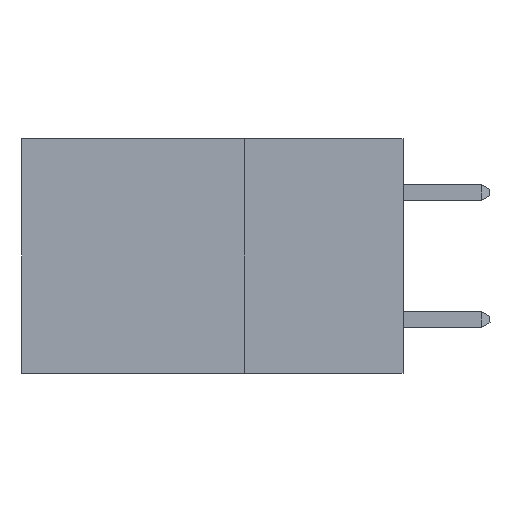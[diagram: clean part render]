
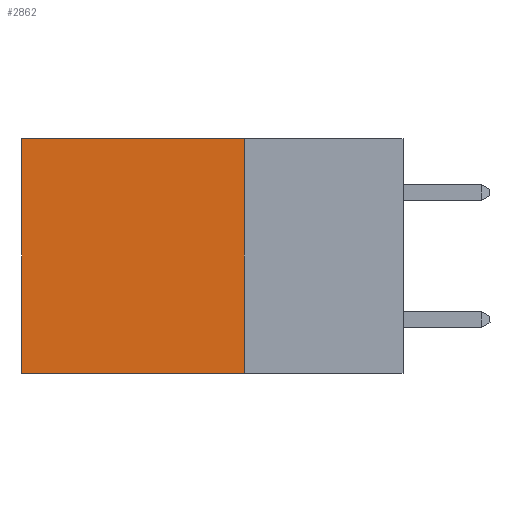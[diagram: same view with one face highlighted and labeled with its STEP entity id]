
A CAD part, left-side view. The second image highlights one B-rep face of the part: STEP entity #2862.
In plain terms, the highlighted planar face has unit normal (-1, 0, 0).
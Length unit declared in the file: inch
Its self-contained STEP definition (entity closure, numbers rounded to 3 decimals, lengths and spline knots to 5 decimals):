
#888 = LINE ( 'NONE', #14398, #5007 ) ;
#1126 = FACE_OUTER_BOUND ( 'NONE', #6531, .T. ) ;
#1230 = DIRECTION ( 'NONE',  ( 0., 0., -1. ) ) ;
#1485 = VERTEX_POINT ( 'NONE', #10861 ) ;
#1692 = LINE ( 'NONE', #4497, #5118 ) ;
#2842 = CARTESIAN_POINT ( 'NONE',  ( 0.2875, 0.25, -0.37 ) ) ;
#2862 = ADVANCED_FACE ( 'NONE', ( #1126 ), #5157, .F. ) ;
#2974 = ORIENTED_EDGE ( 'NONE', *, *, #4944, .T. ) ;
#3837 = CARTESIAN_POINT ( 'NONE',  ( 0.2875, 0.6, 0. ) ) ;
#4074 = DIRECTION ( 'NONE',  ( 0., 1., 0. ) ) ;
#4497 = CARTESIAN_POINT ( 'NONE',  ( 0.2875, 0.25, 0. ) ) ;
#4889 = VERTEX_POINT ( 'NONE', #8731 ) ;
#4944 = EDGE_CURVE ( 'NONE', #5792, #4889, #888, .T. ) ;
#5007 = VECTOR ( 'NONE', #12112, 39.37008 ) ;
#5118 = VECTOR ( 'NONE', #1230, 39.37008 ) ;
#5157 = PLANE ( 'NONE',  #8720 ) ;
#5349 = LINE ( 'NONE', #12323, #13307 ) ;
#5426 = ORIENTED_EDGE ( 'NONE', *, *, #12861, .T. ) ;
#5441 = ORIENTED_EDGE ( 'NONE', *, *, #14549, .F. ) ;
#5792 = VERTEX_POINT ( 'NONE', #3837 ) ;
#6107 = VERTEX_POINT ( 'NONE', #2842 ) ;
#6531 = EDGE_LOOP ( 'NONE', ( #2974, #9003, #5441, #5426 ) ) ;
#7271 = LINE ( 'NONE', #10882, #7634 ) ;
#7555 = DIRECTION ( 'NONE',  ( 1., 0., 0. ) ) ;
#7634 = VECTOR ( 'NONE', #4074, 39.37008 ) ;
#7866 = EDGE_CURVE ( 'NONE', #6107, #4889, #7271, .T. ) ;
#8720 = AXIS2_PLACEMENT_3D ( 'NONE', #12961, #7555, #9868 ) ;
#8731 = CARTESIAN_POINT ( 'NONE',  ( 0.2875, 0.6, -0.37 ) ) ;
#9003 = ORIENTED_EDGE ( 'NONE', *, *, #7866, .F. ) ;
#9868 = DIRECTION ( 'NONE',  ( 0., 0., -1. ) ) ;
#10861 = CARTESIAN_POINT ( 'NONE',  ( 0.2875, 0.25, 0. ) ) ;
#10882 = CARTESIAN_POINT ( 'NONE',  ( 0.2875, 0.25, -0.37 ) ) ;
#12112 = DIRECTION ( 'NONE',  ( 0., 0., -1. ) ) ;
#12323 = CARTESIAN_POINT ( 'NONE',  ( 0.2875, 0.25, 0. ) ) ;
#12861 = EDGE_CURVE ( 'NONE', #1485, #5792, #5349, .T. ) ;
#12961 = CARTESIAN_POINT ( 'NONE',  ( 0.2875, 0.25, 0. ) ) ;
#13307 = VECTOR ( 'NONE', #13433, 39.37008 ) ;
#13433 = DIRECTION ( 'NONE',  ( 0., 1., 0. ) ) ;
#14398 = CARTESIAN_POINT ( 'NONE',  ( 0.2875, 0.6, 0. ) ) ;
#14549 = EDGE_CURVE ( 'NONE', #1485, #6107, #1692, .T. ) ;
